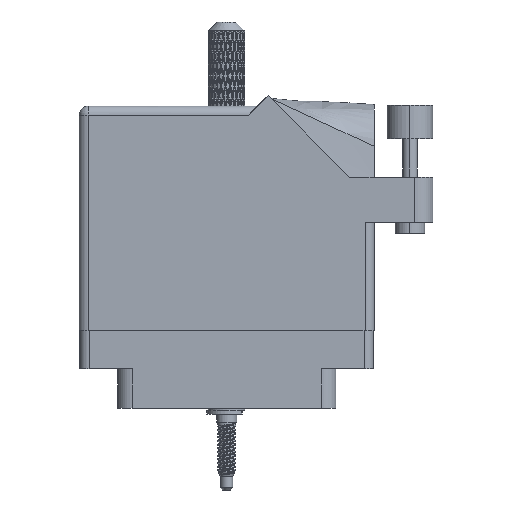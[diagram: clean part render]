
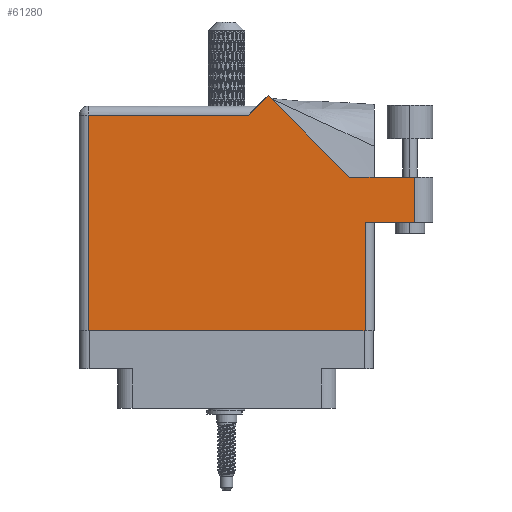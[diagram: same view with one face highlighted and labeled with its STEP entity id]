
A CAD part, front view. The second image highlights one B-rep face of the part: STEP entity #61280.
In plain terms, the highlighted face is planar.
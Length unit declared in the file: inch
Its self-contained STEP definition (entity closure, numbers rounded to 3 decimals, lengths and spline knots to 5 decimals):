
#662 = EDGE_CURVE ( 'NONE', #48689, #87548, #98536, .T. ) ;
#1987 = CARTESIAN_POINT ( 'NONE',  ( 0.062, 1.468, 0. ) ) ;
#2457 = ORIENTED_EDGE ( 'NONE', *, *, #82461, .T. ) ;
#5289 = ORIENTED_EDGE ( 'NONE', *, *, #96179, .T. ) ;
#7078 = LINE ( 'NONE', #24126, #43801 ) ;
#7857 = VERTEX_POINT ( 'NONE', #91684 ) ;
#11213 = CARTESIAN_POINT ( 'NONE',  ( 1.948, 0.737, 0. ) ) ;
#13085 = VERTEX_POINT ( 'NONE', #11213 ) ;
#17030 = DIRECTION ( 'NONE',  ( 0., 1., 0. ) ) ;
#22582 = CARTESIAN_POINT ( 'NONE',  ( 1.948, 0.737, 0. ) ) ;
#23770 = DIRECTION ( 'NONE',  ( -0.707, 0.707, 0. ) ) ;
#24126 = CARTESIAN_POINT ( 'NONE',  ( 1.84442, 1.044, 0. ) ) ;
#24417 = CARTESIAN_POINT ( 'NONE',  ( 2.285, 1.044, 0. ) ) ;
#26357 = ORIENTED_EDGE ( 'NONE', *, *, #87960, .T. ) ;
#29075 = VECTOR ( 'NONE', #39629, 39.37008 ) ;
#29246 = LINE ( 'NONE', #89505, #79902 ) ;
#31408 = DIRECTION ( 'NONE',  ( -1., 0., 0. ) ) ;
#39363 = DIRECTION ( 'NONE',  ( 0., 0., -1. ) ) ;
#39629 = DIRECTION ( 'NONE',  ( -0.707, -0.707, 0. ) ) ;
#39971 = CARTESIAN_POINT ( 'NONE',  ( 1.217, 1.53, 0. ) ) ;
#40223 = CARTESIAN_POINT ( 'NONE',  ( 2.41, 1.044, 0. ) ) ;
#40688 = EDGE_CURVE ( 'NONE', #77704, #85550, #97704, .T. ) ;
#43801 = VECTOR ( 'NONE', #23770, 39.37008 ) ;
#47397 = ORIENTED_EDGE ( 'NONE', *, *, #80287, .T. ) ;
#47505 = CARTESIAN_POINT ( 'NONE',  ( 0.062, 0., 0. ) ) ;
#48689 = VERTEX_POINT ( 'NONE', #64826 ) ;
#49328 = CARTESIAN_POINT ( 'NONE',  ( 2.285, 1.044, 0. ) ) ;
#49364 = DIRECTION ( 'NONE',  ( -1., 0., 0. ) ) ;
#52217 = VECTOR ( 'NONE', #31408, 39.37008 ) ;
#54879 = DIRECTION ( 'NONE',  ( 0., 1., 0. ) ) ;
#55350 = DIRECTION ( 'NONE',  ( 0., -1., 0. ) ) ;
#58581 = ORIENTED_EDGE ( 'NONE', *, *, #74296, .T. ) ;
#58901 = DIRECTION ( 'NONE',  ( 1., 0., 0. ) ) ;
#61280 = ADVANCED_FACE ( 'NONE', ( #94333 ), #63880, .F. ) ;
#62525 = VECTOR ( 'NONE', #54879, 39.37008 ) ;
#62948 = CARTESIAN_POINT ( 'NONE',  ( 0., 1.468, 0. ) ) ;
#63560 = LINE ( 'NONE', #24417, #103839 ) ;
#63880 = PLANE ( 'NONE',  #92909 ) ;
#64826 = CARTESIAN_POINT ( 'NONE',  ( 1.28771, 1.60071, 0. ) ) ;
#66237 = LINE ( 'NONE', #22582, #62525 ) ;
#70946 = LINE ( 'NONE', #98616, #84765 ) ;
#71127 = ORIENTED_EDGE ( 'NONE', *, *, #72528, .T. ) ;
#72528 = EDGE_CURVE ( 'NONE', #102807, #13085, #66237, .T. ) ;
#73178 = LINE ( 'NONE', #62948, #79472 ) ;
#74296 = EDGE_CURVE ( 'NONE', #102475, #83592, #63560, .T. ) ;
#76273 = ORIENTED_EDGE ( 'NONE', *, *, #40688, .T. ) ;
#76366 = VECTOR ( 'NONE', #55350, 39.37008 ) ;
#76837 = CARTESIAN_POINT ( 'NONE',  ( 0.062, 0., 0. ) ) ;
#77704 = VERTEX_POINT ( 'NONE', #1987 ) ;
#79472 = VECTOR ( 'NONE', #49364, 39.37008 ) ;
#79902 = VECTOR ( 'NONE', #98298, 39.37008 ) ;
#80287 = EDGE_CURVE ( 'NONE', #87548, #77704, #73178, .T. ) ;
#80389 = DIRECTION ( 'NONE',  ( -1., 0., 0. ) ) ;
#82461 = EDGE_CURVE ( 'NONE', #13085, #102475, #29246, .T. ) ;
#83064 = ORIENTED_EDGE ( 'NONE', *, *, #92636, .T. ) ;
#83592 = VERTEX_POINT ( 'NONE', #49328 ) ;
#83727 = CARTESIAN_POINT ( 'NONE',  ( 1.155, 1.468, 0. ) ) ;
#84765 = VECTOR ( 'NONE', #58901, 39.37008 ) ;
#85550 = VERTEX_POINT ( 'NONE', #76837 ) ;
#86113 = ORIENTED_EDGE ( 'NONE', *, *, #662, .T. ) ;
#87548 = VERTEX_POINT ( 'NONE', #83727 ) ;
#87960 = EDGE_CURVE ( 'NONE', #85550, #102807, #70946, .T. ) ;
#89505 = CARTESIAN_POINT ( 'NONE',  ( 2.01, 0.737, 0. ) ) ;
#91684 = CARTESIAN_POINT ( 'NONE',  ( 1.84442, 1.044, 0. ) ) ;
#92636 = EDGE_CURVE ( 'NONE', #7857, #48689, #7078, .T. ) ;
#92909 = AXIS2_PLACEMENT_3D ( 'NONE', #96170, #39363, #80389 ) ;
#94333 = FACE_OUTER_BOUND ( 'NONE', #98502, .T. ) ;
#96170 = CARTESIAN_POINT ( 'NONE',  ( 0., 1.53, 0. ) ) ;
#96179 = EDGE_CURVE ( 'NONE', #83592, #7857, #102719, .T. ) ;
#97704 = LINE ( 'NONE', #47505, #76366 ) ;
#98298 = DIRECTION ( 'NONE',  ( 1., 0., 0. ) ) ;
#98502 = EDGE_LOOP ( 'NONE', ( #2457, #58581, #5289, #83064, #86113, #47397, #76273, #26357, #71127 ) ) ;
#98536 = LINE ( 'NONE', #39971, #29075 ) ;
#98616 = CARTESIAN_POINT ( 'NONE',  ( 0., 0., 0. ) ) ;
#98620 = CARTESIAN_POINT ( 'NONE',  ( 1.948, 0., 0. ) ) ;
#99784 = CARTESIAN_POINT ( 'NONE',  ( 2.285, 0.737, 0. ) ) ;
#102475 = VERTEX_POINT ( 'NONE', #99784 ) ;
#102719 = LINE ( 'NONE', #40223, #52217 ) ;
#102807 = VERTEX_POINT ( 'NONE', #98620 ) ;
#103839 = VECTOR ( 'NONE', #17030, 39.37008 ) ;
